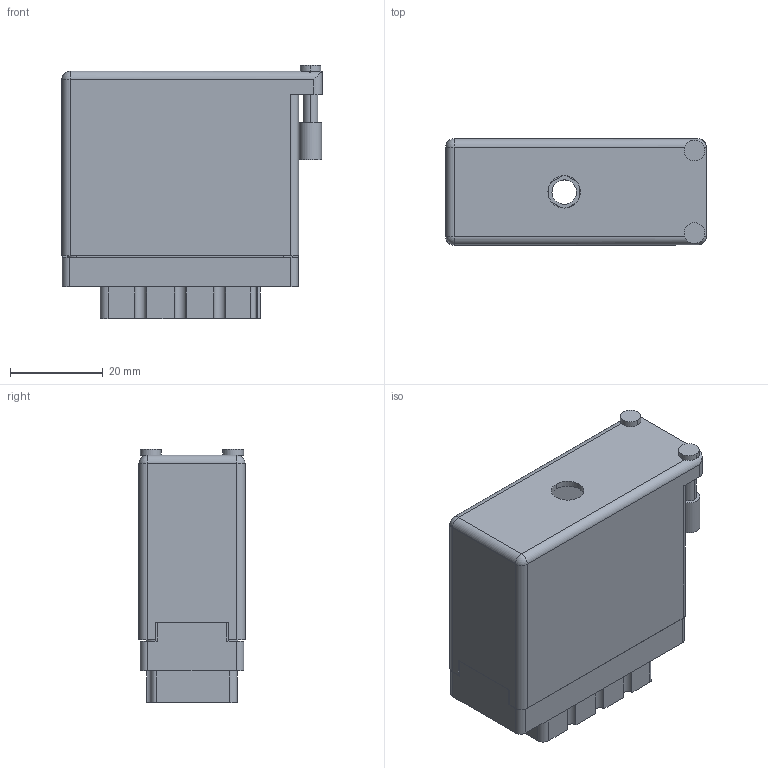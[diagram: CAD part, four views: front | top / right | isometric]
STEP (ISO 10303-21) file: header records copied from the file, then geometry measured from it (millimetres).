
FILE_DESCRIPTION (( 'STEP AP203' ), '1' );
FILE_NAME ('516-038-000-250.STEP', '2020-03-04T21:32:11', ( '' ), ( '' ), 'SwSTEP 2.0', 'SolidWorks 2016', '' );
FILE_SCHEMA (( 'CONFIG_CONTROL_DESIGN' ));
Length unit declared in the file: inch
Products named in the file (3): 516-038-000-250; 516 Part Receptacle_038; 516-230-001_Metal - 038 Side Entry
Assembly tree (2 placements, depth 2):
  516-038-000-250
    516 Part Receptacle_038
    516-230-001_Metal - 038 Side Entry
Bounding box: 56.08 x 22.83 x 54.53 mm (x, y, z)
Volume: 19368.2 mm3; surface area: 28004.7 mm2
Topology: 2 solids, 2 shells, 979 faces, 2863 edges, 1902 vertices
Faces by surface type: plane 670, cylinder 305, cone 2, sphere 2
Entity records: 32999 total; most frequent: CARTESIAN_POINT 5788, ORIENTED_EDGE 5722, DIRECTION 5584, EDGE_CURVE 2861, VECTOR 2096, LINE 2096, VERTEX_POINT 1902, AXIS2_PLACEMENT_3D 1744
